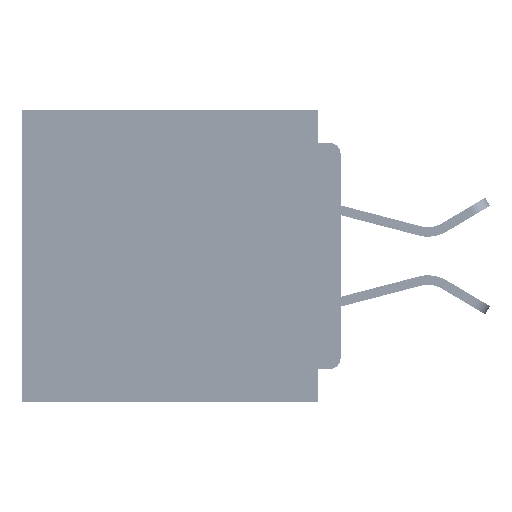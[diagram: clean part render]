
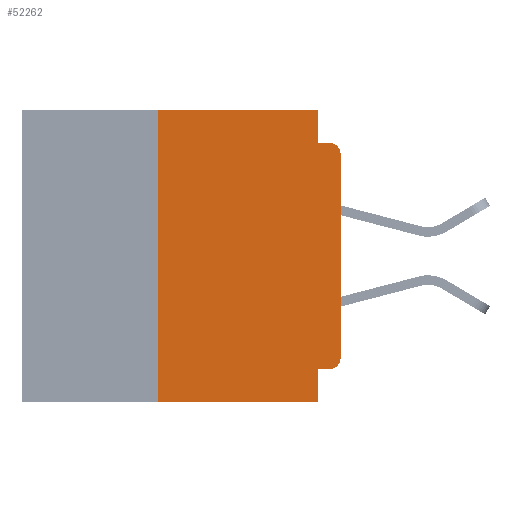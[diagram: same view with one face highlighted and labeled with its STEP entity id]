
A CAD part, left-side view. The second image highlights one B-rep face of the part: STEP entity #52262.
In plain terms, the highlighted planar face has unit normal (-1, 0, 0).
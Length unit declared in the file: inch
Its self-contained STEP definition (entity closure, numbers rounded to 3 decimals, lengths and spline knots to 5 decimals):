
#57 = DIRECTION ( 'NONE',  ( 0., -1., 0. ) ) ;
#2401 = DIRECTION ( 'NONE',  ( 0., -1., 0. ) ) ;
#5640 = ORIENTED_EDGE ( 'NONE', *, *, #21536, .T. ) ;
#6518 = LINE ( 'NONE', #56593, #42694 ) ;
#6806 = CARTESIAN_POINT ( 'NONE',  ( 0., 0., -0.34 ) ) ;
#7118 = LINE ( 'NONE', #19516, #18141 ) ;
#7217 = CARTESIAN_POINT ( 'NONE',  ( 0., 0.437, 0. ) ) ;
#8607 = CARTESIAN_POINT ( 'NONE',  ( 0., 0.015, -0.06 ) ) ;
#11499 = VECTOR ( 'NONE', #17033, 39.37008 ) ;
#12972 = LINE ( 'NONE', #45375, #11499 ) ;
#13335 = DIRECTION ( 'NONE',  ( 0., 0., -1. ) ) ;
#14827 = VERTEX_POINT ( 'NONE', #20973 ) ;
#15085 = CARTESIAN_POINT ( 'NONE',  ( 0., 0.031, -0.4 ) ) ;
#15089 = DIRECTION ( 'NONE',  ( 0., 0., 1. ) ) ;
#15710 = CARTESIAN_POINT ( 'NONE',  ( 0., 0.437, -0.4 ) ) ;
#16657 = DIRECTION ( 'NONE',  ( 1., 0., 0. ) ) ;
#16856 = FACE_OUTER_BOUND ( 'NONE', #53932, .T. ) ;
#17033 = DIRECTION ( 'NONE',  ( 0., 0., -1. ) ) ;
#18141 = VECTOR ( 'NONE', #57266, 39.37008 ) ;
#19016 = LINE ( 'NONE', #15710, #41209 ) ;
#19022 = VERTEX_POINT ( 'NONE', #15085 ) ;
#19516 = CARTESIAN_POINT ( 'NONE',  ( 0., 0.031, 0. ) ) ;
#20973 = CARTESIAN_POINT ( 'NONE',  ( 0., 0., -0.06 ) ) ;
#21183 = EDGE_CURVE ( 'NONE', #44870, #56122, #22811, .T. ) ;
#21231 = PLANE ( 'NONE',  #48543 ) ;
#21536 = EDGE_CURVE ( 'NONE', #58979, #30495, #36792, .T. ) ;
#22127 = EDGE_CURVE ( 'NONE', #30495, #14827, #40402, .T. ) ;
#22509 = CARTESIAN_POINT ( 'NONE',  ( 0., 0.031, 0. ) ) ;
#22558 = EDGE_CURVE ( 'NONE', #25356, #26837, #54358, .T. ) ;
#22811 = LINE ( 'NONE', #29142, #32415 ) ;
#25356 = VERTEX_POINT ( 'NONE', #51517 ) ;
#26590 = LINE ( 'NONE', #52138, #50265 ) ;
#26837 = VERTEX_POINT ( 'NONE', #48545 ) ;
#27019 = DIRECTION ( 'NONE',  ( -1., 0., 0. ) ) ;
#27508 = CIRCLE ( 'NONE', #41570, 0.015 ) ;
#27753 = VECTOR ( 'NONE', #2401, 39.37008 ) ;
#28575 = EDGE_CURVE ( 'NONE', #56122, #59626, #6518, .T. ) ;
#29142 = CARTESIAN_POINT ( 'NONE',  ( 0., 0.25, -0.4 ) ) ;
#30495 = VERTEX_POINT ( 'NONE', #6806 ) ;
#32315 = ORIENTED_EDGE ( 'NONE', *, *, #56433, .T. ) ;
#32415 = VECTOR ( 'NONE', #15089, 39.37008 ) ;
#34864 = CARTESIAN_POINT ( 'NONE',  ( 0., 0.25, 0. ) ) ;
#35703 = CARTESIAN_POINT ( 'NONE',  ( 0., 0.031, -0.355 ) ) ;
#36792 = CIRCLE ( 'NONE', #45693, 0.015 ) ;
#37599 = ORIENTED_EDGE ( 'NONE', *, *, #22558, .F. ) ;
#40168 = CARTESIAN_POINT ( 'NONE',  ( 0., 0., -0.045 ) ) ;
#40402 = LINE ( 'NONE', #41676, #51498 ) ;
#41209 = VECTOR ( 'NONE', #44054, 39.37008 ) ;
#41570 = AXIS2_PLACEMENT_3D ( 'NONE', #8607, #41660, #13335 ) ;
#41660 = DIRECTION ( 'NONE',  ( -1., 0., 0. ) ) ;
#41676 = CARTESIAN_POINT ( 'NONE',  ( 0., 0., 0. ) ) ;
#41948 = VERTEX_POINT ( 'NONE', #35703 ) ;
#42694 = VECTOR ( 'NONE', #57, 39.37008 ) ;
#44004 = CARTESIAN_POINT ( 'NONE',  ( 0., 0.25, -0.4 ) ) ;
#44054 = DIRECTION ( 'NONE',  ( 0., -1., 0. ) ) ;
#44178 = ORIENTED_EDGE ( 'NONE', *, *, #49241, .F. ) ;
#44870 = VERTEX_POINT ( 'NONE', #44004 ) ;
#45375 = CARTESIAN_POINT ( 'NONE',  ( 0., 0.031, -0.4 ) ) ;
#45693 = AXIS2_PLACEMENT_3D ( 'NONE', #55312, #27019, #60020 ) ;
#45755 = CARTESIAN_POINT ( 'NONE',  ( 0., 0.015, -0.355 ) ) ;
#46425 = ORIENTED_EDGE ( 'NONE', *, *, #60554, .F. ) ;
#46445 = DIRECTION ( 'NONE',  ( 0., 0., 1. ) ) ;
#48256 = EDGE_CURVE ( 'NONE', #44870, #19022, #19016, .T. ) ;
#48543 = AXIS2_PLACEMENT_3D ( 'NONE', #7217, #16657, #49739 ) ;
#48545 = CARTESIAN_POINT ( 'NONE',  ( 0., 0.015, -0.045 ) ) ;
#48959 = ORIENTED_EDGE ( 'NONE', *, *, #48256, .T. ) ;
#49241 = EDGE_CURVE ( 'NONE', #41948, #19022, #12972, .T. ) ;
#49739 = DIRECTION ( 'NONE',  ( 0., 0., -1. ) ) ;
#50265 = VECTOR ( 'NONE', #56856, 39.37008 ) ;
#51403 = EDGE_CURVE ( 'NONE', #58979, #41948, #26590, .T. ) ;
#51498 = VECTOR ( 'NONE', #46445, 39.37008 ) ;
#51517 = CARTESIAN_POINT ( 'NONE',  ( 0., 0.031, -0.045 ) ) ;
#52138 = CARTESIAN_POINT ( 'NONE',  ( 0., 0., -0.355 ) ) ;
#52262 = ADVANCED_FACE ( 'NONE', ( #16856 ), #21231, .F. ) ;
#53932 = EDGE_LOOP ( 'NONE', ( #57170, #32315, #37599, #46425, #58886, #58891, #48959, #44178, #57787, #5640 ) ) ;
#54358 = LINE ( 'NONE', #40168, #27753 ) ;
#55312 = CARTESIAN_POINT ( 'NONE',  ( 0., 0.015, -0.34 ) ) ;
#56122 = VERTEX_POINT ( 'NONE', #34864 ) ;
#56433 = EDGE_CURVE ( 'NONE', #14827, #26837, #27508, .T. ) ;
#56593 = CARTESIAN_POINT ( 'NONE',  ( 0., 0.437, 0. ) ) ;
#56856 = DIRECTION ( 'NONE',  ( 0., 1., 0. ) ) ;
#57170 = ORIENTED_EDGE ( 'NONE', *, *, #22127, .T. ) ;
#57266 = DIRECTION ( 'NONE',  ( 0., 0., -1. ) ) ;
#57787 = ORIENTED_EDGE ( 'NONE', *, *, #51403, .F. ) ;
#58886 = ORIENTED_EDGE ( 'NONE', *, *, #28575, .F. ) ;
#58891 = ORIENTED_EDGE ( 'NONE', *, *, #21183, .F. ) ;
#58979 = VERTEX_POINT ( 'NONE', #45755 ) ;
#59626 = VERTEX_POINT ( 'NONE', #22509 ) ;
#60020 = DIRECTION ( 'NONE',  ( 0., 0., -1. ) ) ;
#60554 = EDGE_CURVE ( 'NONE', #59626, #25356, #7118, .T. ) ;
